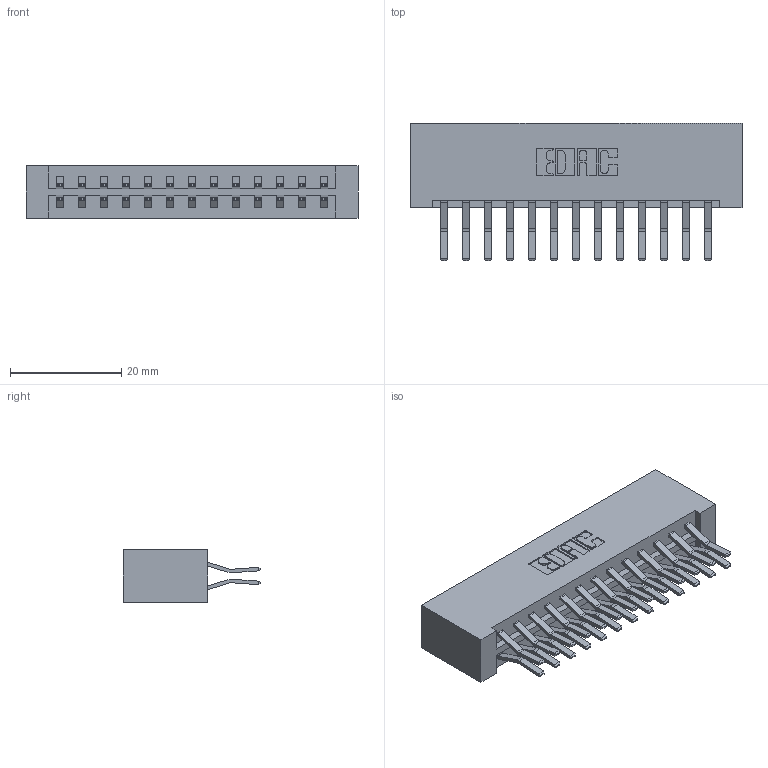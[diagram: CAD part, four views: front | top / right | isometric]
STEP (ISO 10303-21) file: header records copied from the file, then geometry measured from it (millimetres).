
FILE_DESCRIPTION (( 'STEP AP203' ), '1' );
FILE_NAME ('833-026-560-201.STEP', '2020-06-02T05:57:43', ( '' ), ( '' ), 'SwSTEP 2.0', 'SolidWorks 2020', '' );
FILE_SCHEMA (( 'CONFIG_CONTROL_DESIGN' ));
Length unit declared in the file: inch
Products named in the file (3): 833-026-560-201; 345-292-001_560 Tail; 833 Part_Lugless
Assembly tree (27 placements, depth 2):
  833-026-560-201
    833 Part_Lugless
    345-292-001_560 Tail  x26
Bounding box: 59.77 x 24.78 x 9.4 mm (x, y, z)
Volume: 6633.2 mm3; surface area: 8041 mm2
Topology: 27 solids, 27 shells, 1510 faces, 4473 edges, 2946 vertices
Faces by surface type: plane 1002, cylinder 508
Entity records: 11925 total; most frequent: CARTESIAN_POINT 2010, ORIENTED_EDGE 1946, DIRECTION 1765, EDGE_CURVE 973, LINE 849, VECTOR 849, VERTEX_POINT 646, AXIS2_PLACEMENT_3D 458
